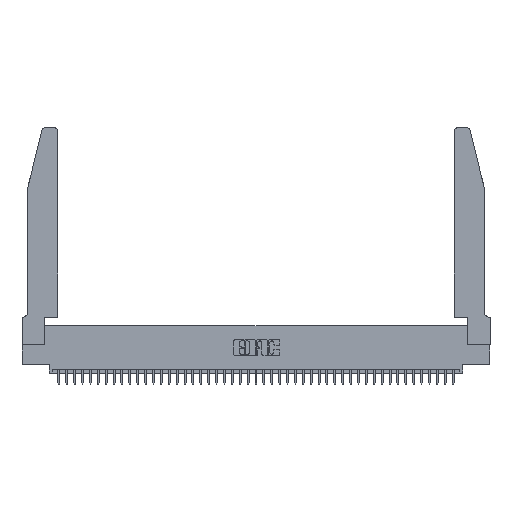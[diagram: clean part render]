
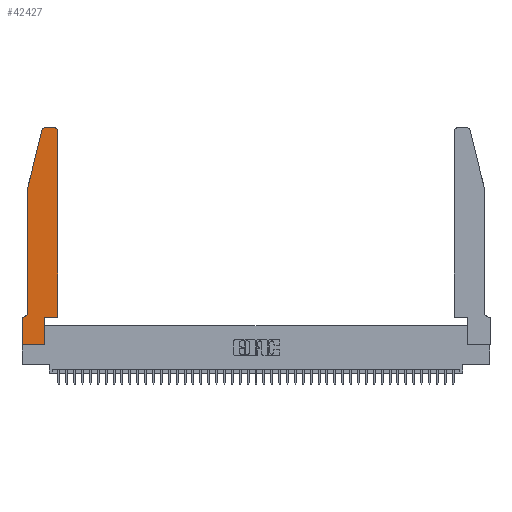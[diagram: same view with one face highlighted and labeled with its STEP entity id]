
A CAD part, top view. The second image highlights one B-rep face of the part: STEP entity #42427.
In plain terms, the highlighted planar face has unit normal (0, 0, 1).
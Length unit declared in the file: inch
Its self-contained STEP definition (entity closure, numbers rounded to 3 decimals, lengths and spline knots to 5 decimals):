
#43 = EDGE_CURVE ( 'NONE', #34715, #274, #26961, .T. ) ;
#274 = VERTEX_POINT ( 'NONE', #14675 ) ;
#953 = VECTOR ( 'NONE', #5916, 39.37008 ) ;
#1393 = LINE ( 'NONE', #39434, #39461 ) ;
#1707 = CARTESIAN_POINT ( 'NONE',  ( 0.4205, 2.75, 0.37 ) ) ;
#2259 = CARTESIAN_POINT ( 'NONE',  ( 0.0755, 2., 0.37 ) ) ;
#3292 = CARTESIAN_POINT ( 'NONE',  ( 0.4505, 0.35, 0.37 ) ) ;
#3754 = EDGE_CURVE ( 'NONE', #30532, #7736, #11082, .T. ) ;
#3771 = ORIENTED_EDGE ( 'NONE', *, *, #16653, .T. ) ;
#3889 = ORIENTED_EDGE ( 'NONE', *, *, #3754, .T. ) ;
#4422 = ORIENTED_EDGE ( 'NONE', *, *, #7698, .T. ) ;
#5657 = DIRECTION ( 'NONE',  ( -0.239, -0.971, 0. ) ) ;
#5916 = DIRECTION ( 'NONE',  ( 0., -1., 0. ) ) ;
#6009 = ORIENTED_EDGE ( 'NONE', *, *, #43422, .T. ) ;
#6045 = VERTEX_POINT ( 'NONE', #24595 ) ;
#6089 = AXIS2_PLACEMENT_3D ( 'NONE', #37815, #17650, #41184 ) ;
#6437 = VECTOR ( 'NONE', #38477, 39.37008 ) ;
#7698 = EDGE_CURVE ( 'NONE', #7736, #38424, #8637, .T. ) ;
#7736 = VERTEX_POINT ( 'NONE', #16341 ) ;
#7903 = CARTESIAN_POINT ( 'NONE',  ( 0.284, 2.75, 0.37 ) ) ;
#8429 = VERTEX_POINT ( 'NONE', #3292 ) ;
#8637 = CIRCLE ( 'NONE', #27553, 0.07 ) ;
#9631 = CARTESIAN_POINT ( 'NONE',  ( 0.0055, 0.35, 0.37 ) ) ;
#9909 = DIRECTION ( 'NONE',  ( 1., 0., 0. ) ) ;
#10584 = VERTEX_POINT ( 'NONE', #1707 ) ;
#11082 = LINE ( 'NONE', #39565, #953 ) ;
#11300 = AXIS2_PLACEMENT_3D ( 'NONE', #20205, #43690, #23570 ) ;
#11989 = EDGE_CURVE ( 'NONE', #31411, #24017, #18032, .T. ) ;
#12412 = ORIENTED_EDGE ( 'NONE', *, *, #11989, .T. ) ;
#12636 = ORIENTED_EDGE ( 'NONE', *, *, #43, .T. ) ;
#12836 = DIRECTION ( 'NONE',  ( 0., 0., -1. ) ) ;
#14338 = VECTOR ( 'NONE', #16368, 39.37008 ) ;
#14570 = LINE ( 'NONE', #33497, #40412 ) ;
#14675 = CARTESIAN_POINT ( 'NONE',  ( 0.25487, 2.72718, 0.37 ) ) ;
#15005 = ORIENTED_EDGE ( 'NONE', *, *, #40886, .T. ) ;
#15325 = CARTESIAN_POINT ( 'NONE',  ( 0., 0.35, 0.37 ) ) ;
#15716 = CARTESIAN_POINT ( 'NONE',  ( 0.4505, 2.72, 0.37 ) ) ;
#16341 = CARTESIAN_POINT ( 'NONE',  ( 0.0755, 0.42, 0.37 ) ) ;
#16368 = DIRECTION ( 'NONE',  ( -1., 0., 0. ) ) ;
#16653 = EDGE_CURVE ( 'NONE', #10584, #34715, #1393, .T. ) ;
#17622 = FACE_OUTER_BOUND ( 'NONE', #30855, .T. ) ;
#17650 = DIRECTION ( 'NONE',  ( 0., 0., 1. ) ) ;
#17840 = ORIENTED_EDGE ( 'NONE', *, *, #18617, .T. ) ;
#17943 = DIRECTION ( 'NONE',  ( 0., 0., 1. ) ) ;
#18032 = LINE ( 'NONE', #36216, #25918 ) ;
#18038 = VECTOR ( 'NONE', #40031, 39.37008 ) ;
#18617 = EDGE_CURVE ( 'NONE', #274, #30532, #36127, .T. ) ;
#19284 = DIRECTION ( 'NONE',  ( -1., 0., 0. ) ) ;
#19810 = EDGE_CURVE ( 'NONE', #8429, #33566, #32320, .T. ) ;
#20179 = LINE ( 'NONE', #36655, #18038 ) ;
#20205 = CARTESIAN_POINT ( 'NONE',  ( 0.284, 2.72, 0.37 ) ) ;
#21510 = CARTESIAN_POINT ( 'NONE',  ( 0.2865, 0., 0.37 ) ) ;
#21722 = CARTESIAN_POINT ( 'NONE',  ( 0.4505, 0.35, 0.37 ) ) ;
#22613 = CARTESIAN_POINT ( 'NONE',  ( 0.4505, 0.35, 0.37 ) ) ;
#23304 = CIRCLE ( 'NONE', #6089, 0.03 ) ;
#23570 = DIRECTION ( 'NONE',  ( 1., 0., 0. ) ) ;
#24017 = VERTEX_POINT ( 'NONE', #27037 ) ;
#24595 = CARTESIAN_POINT ( 'NONE',  ( 0.2865, 0.35, 0.37 ) ) ;
#25412 = LINE ( 'NONE', #22613, #42249 ) ;
#25918 = VECTOR ( 'NONE', #39606, 39.37008 ) ;
#26279 = EDGE_CURVE ( 'NONE', #6045, #8429, #25412, .T. ) ;
#26886 = CARTESIAN_POINT ( 'NONE',  ( 0.0755, 2., 0.37 ) ) ;
#26961 = CIRCLE ( 'NONE', #11300, 0.03 ) ;
#27037 = CARTESIAN_POINT ( 'NONE',  ( 0., 0., 0.37 ) ) ;
#27139 = ORIENTED_EDGE ( 'NONE', *, *, #33703, .T. ) ;
#27553 = AXIS2_PLACEMENT_3D ( 'NONE', #33008, #12836, #36401 ) ;
#29367 = DIRECTION ( 'NONE',  ( 1., 0., 0. ) ) ;
#29819 = ORIENTED_EDGE ( 'NONE', *, *, #26279, .T. ) ;
#30153 = VERTEX_POINT ( 'NONE', #21510 ) ;
#30284 = ORIENTED_EDGE ( 'NONE', *, *, #19810, .T. ) ;
#30532 = VERTEX_POINT ( 'NONE', #26886 ) ;
#30855 = EDGE_LOOP ( 'NONE', ( #3771, #12636, #17840, #3889, #4422, #6009, #12412, #15005, #27139, #29819, #30284, #35619 ) ) ;
#31340 = PLANE ( 'NONE',  #36738 ) ;
#31411 = VERTEX_POINT ( 'NONE', #15325 ) ;
#32320 = LINE ( 'NONE', #21722, #6437 ) ;
#33008 = CARTESIAN_POINT ( 'NONE',  ( 0.0055, 0.42, 0.37 ) ) ;
#33349 = LINE ( 'NONE', #36568, #14338 ) ;
#33497 = CARTESIAN_POINT ( 'NONE',  ( 0., 0., 0.37 ) ) ;
#33566 = VERTEX_POINT ( 'NONE', #15716 ) ;
#33703 = EDGE_CURVE ( 'NONE', #30153, #6045, #20179, .T. ) ;
#34715 = VERTEX_POINT ( 'NONE', #7903 ) ;
#35068 = VECTOR ( 'NONE', #5657, 39.37008 ) ;
#35619 = ORIENTED_EDGE ( 'NONE', *, *, #37969, .T. ) ;
#36127 = LINE ( 'NONE', #2259, #35068 ) ;
#36216 = CARTESIAN_POINT ( 'NONE',  ( 0., 0., 0.37 ) ) ;
#36401 = DIRECTION ( 'NONE',  ( -1., 0., 0. ) ) ;
#36568 = CARTESIAN_POINT ( 'NONE',  ( 0.0755, 0.35, 0.37 ) ) ;
#36655 = CARTESIAN_POINT ( 'NONE',  ( 0.2865, 0.35, 0.37 ) ) ;
#36738 = AXIS2_PLACEMENT_3D ( 'NONE', #38109, #17943, #41482 ) ;
#37815 = CARTESIAN_POINT ( 'NONE',  ( 0.4205, 2.72, 0.37 ) ) ;
#37969 = EDGE_CURVE ( 'NONE', #33566, #10584, #23304, .T. ) ;
#38109 = CARTESIAN_POINT ( 'NONE',  ( 0., 0.35, 0.37 ) ) ;
#38424 = VERTEX_POINT ( 'NONE', #9631 ) ;
#38477 = DIRECTION ( 'NONE',  ( 0., 1., 0. ) ) ;
#39434 = CARTESIAN_POINT ( 'NONE',  ( 0.2605, 2.75, 0.37 ) ) ;
#39461 = VECTOR ( 'NONE', #19284, 39.37008 ) ;
#39565 = CARTESIAN_POINT ( 'NONE',  ( 0.0755, 2., 0.37 ) ) ;
#39606 = DIRECTION ( 'NONE',  ( 0., -1., 0. ) ) ;
#40031 = DIRECTION ( 'NONE',  ( 0., 1., 0. ) ) ;
#40412 = VECTOR ( 'NONE', #9909, 39.37008 ) ;
#40886 = EDGE_CURVE ( 'NONE', #24017, #30153, #14570, .T. ) ;
#41184 = DIRECTION ( 'NONE',  ( 1., 0., 0. ) ) ;
#41482 = DIRECTION ( 'NONE',  ( 1., 0., 0. ) ) ;
#42249 = VECTOR ( 'NONE', #29367, 39.37008 ) ;
#42427 = ADVANCED_FACE ( 'NONE', ( #17622 ), #31340, .T. ) ;
#43422 = EDGE_CURVE ( 'NONE', #38424, #31411, #33349, .T. ) ;
#43690 = DIRECTION ( 'NONE',  ( 0., 0., 1. ) ) ;
